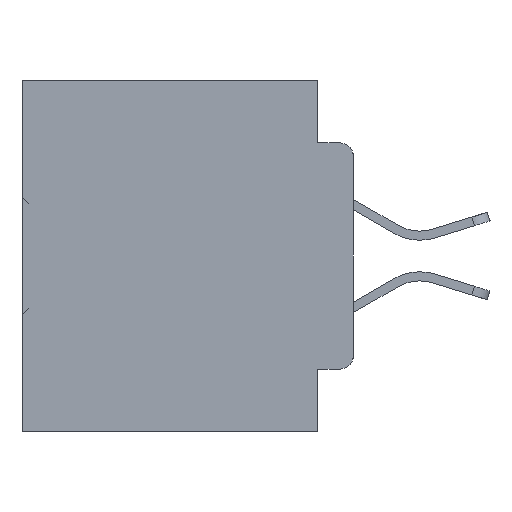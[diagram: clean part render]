
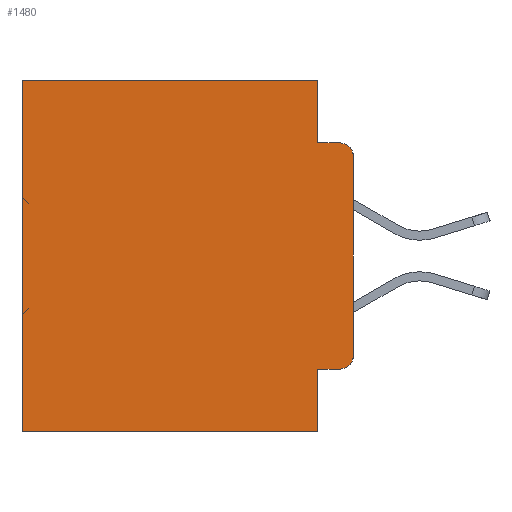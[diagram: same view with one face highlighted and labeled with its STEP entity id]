
A CAD part, left-side view. The second image highlights one B-rep face of the part: STEP entity #1480.
In plain terms, the highlighted planar face has unit normal (-1, 0, 0).
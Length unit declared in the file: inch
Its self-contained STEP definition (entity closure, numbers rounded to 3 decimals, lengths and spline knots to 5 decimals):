
#764 = CARTESIAN_POINT ( 'NONE',  ( 0.298, 0.02, -0.1085 ) ) ;
#821 = DIRECTION ( 'NONE',  ( 0., 1., 0. ) ) ;
#1219 = LINE ( 'NONE', #12970, #22932 ) ;
#1480 = ADVANCED_FACE ( 'NONE', ( #25447 ), #25645, .F. ) ;
#1769 = DIRECTION ( 'NONE',  ( 0., 0., -1. ) ) ;
#2023 = LINE ( 'NONE', #35336, #12925 ) ;
#2050 = CARTESIAN_POINT ( 'NONE',  ( 0.298, 0.051, -0.0885 ) ) ;
#2402 = CARTESIAN_POINT ( 'NONE',  ( 0.298, 0., -0.3915 ) ) ;
#3881 = VECTOR ( 'NONE', #14448, 39.37008 ) ;
#4180 = VECTOR ( 'NONE', #821, 39.37008 ) ;
#4468 = CARTESIAN_POINT ( 'NONE',  ( 0.298, 0.051, 0. ) ) ;
#5771 = LINE ( 'NONE', #36107, #29802 ) ;
#6191 = EDGE_CURVE ( 'NONE', #25917, #34526, #17168, .T. ) ;
#6485 = CARTESIAN_POINT ( 'NONE',  ( 0.298, 0.051, 0. ) ) ;
#7888 = ORIENTED_EDGE ( 'NONE', *, *, #6191, .F. ) ;
#8246 = VECTOR ( 'NONE', #15676, 39.37008 ) ;
#8309 = ORIENTED_EDGE ( 'NONE', *, *, #28857, .T. ) ;
#8771 = AXIS2_PLACEMENT_3D ( 'NONE', #764, #18760, #27748 ) ;
#8822 = AXIS2_PLACEMENT_3D ( 'NONE', #14044, #13656, #25971 ) ;
#8864 = LINE ( 'NONE', #30186, #8246 ) ;
#9851 = ORIENTED_EDGE ( 'NONE', *, *, #35419, .F. ) ;
#9973 = CARTESIAN_POINT ( 'NONE',  ( 0.298, 0.02, -0.0885 ) ) ;
#11407 = EDGE_CURVE ( 'NONE', #37395, #28947, #2023, .T. ) ;
#11568 = EDGE_CURVE ( 'NONE', #28137, #36050, #5771, .T. ) ;
#11791 = CARTESIAN_POINT ( 'NONE',  ( 0.298, 0., -0.1085 ) ) ;
#11933 = CIRCLE ( 'NONE', #8822, 0.02 ) ;
#12596 = DIRECTION ( 'NONE',  ( 0., -1., 0. ) ) ;
#12925 = VECTOR ( 'NONE', #29259, 39.37008 ) ;
#12970 = CARTESIAN_POINT ( 'NONE',  ( 0.298, 0.051, -0.4115 ) ) ;
#13656 = DIRECTION ( 'NONE',  ( -1., 0., 0. ) ) ;
#13900 = CARTESIAN_POINT ( 'NONE',  ( 0.298, 0.051, -0.4115 ) ) ;
#14044 = CARTESIAN_POINT ( 'NONE',  ( 0.298, 0.02, -0.3915 ) ) ;
#14448 = DIRECTION ( 'NONE',  ( 0., 0., -1. ) ) ;
#14636 = EDGE_LOOP ( 'NONE', ( #35437, #30565, #36561, #21337, #8309, #20432, #9851, #7888, #35831, #35888 ) ) ;
#15676 = DIRECTION ( 'NONE',  ( 0., 1., 0. ) ) ;
#15684 = LINE ( 'NONE', #36489, #4180 ) ;
#15830 = EDGE_CURVE ( 'NONE', #19145, #28137, #20118, .T. ) ;
#16073 = DIRECTION ( 'NONE',  ( 0., -1., 0. ) ) ;
#16640 = CARTESIAN_POINT ( 'NONE',  ( 0.298, 0., 0. ) ) ;
#17168 = LINE ( 'NONE', #25973, #3881 ) ;
#18032 = EDGE_CURVE ( 'NONE', #31664, #37157, #37619, .T. ) ;
#18760 = DIRECTION ( 'NONE',  ( -1., 0., 0. ) ) ;
#19145 = VERTEX_POINT ( 'NONE', #6485 ) ;
#20118 = LINE ( 'NONE', #4468, #26246 ) ;
#20432 = ORIENTED_EDGE ( 'NONE', *, *, #11407, .T. ) ;
#21337 = ORIENTED_EDGE ( 'NONE', *, *, #15830, .F. ) ;
#21567 = VERTEX_POINT ( 'NONE', #35968 ) ;
#21885 = CIRCLE ( 'NONE', #8771, 0.02 ) ;
#22683 = DIRECTION ( 'NONE',  ( 0., 0., -1. ) ) ;
#22932 = VECTOR ( 'NONE', #16073, 39.37008 ) ;
#25447 = FACE_OUTER_BOUND ( 'NONE', #14636, .T. ) ;
#25645 = PLANE ( 'NONE',  #27713 ) ;
#25917 = VERTEX_POINT ( 'NONE', #13900 ) ;
#25971 = DIRECTION ( 'NONE',  ( 0., 0., -1. ) ) ;
#25973 = CARTESIAN_POINT ( 'NONE',  ( 0.298, 0.051, 0. ) ) ;
#26246 = VECTOR ( 'NONE', #34632, 39.37008 ) ;
#26335 = EDGE_CURVE ( 'NONE', #31664, #36050, #21885, .T. ) ;
#27713 = AXIS2_PLACEMENT_3D ( 'NONE', #16640, #28597, #1769 ) ;
#27748 = DIRECTION ( 'NONE',  ( 0., 0., -1. ) ) ;
#28137 = VERTEX_POINT ( 'NONE', #2050 ) ;
#28597 = DIRECTION ( 'NONE',  ( 1., 0., 0. ) ) ;
#28803 = CARTESIAN_POINT ( 'NONE',  ( 0.298, 0.473, -0.5 ) ) ;
#28857 = EDGE_CURVE ( 'NONE', #19145, #37395, #15684, .T. ) ;
#28947 = VERTEX_POINT ( 'NONE', #28803 ) ;
#29259 = DIRECTION ( 'NONE',  ( 0., 0., -1. ) ) ;
#29802 = VECTOR ( 'NONE', #12596, 39.37008 ) ;
#30167 = EDGE_CURVE ( 'NONE', #25917, #21567, #1219, .T. ) ;
#30186 = CARTESIAN_POINT ( 'NONE',  ( 0.298, 0., -0.5 ) ) ;
#30317 = VECTOR ( 'NONE', #22683, 39.37008 ) ;
#30565 = ORIENTED_EDGE ( 'NONE', *, *, #26335, .T. ) ;
#31664 = VERTEX_POINT ( 'NONE', #11791 ) ;
#34526 = VERTEX_POINT ( 'NONE', #35455 ) ;
#34632 = DIRECTION ( 'NONE',  ( 0., 0., -1. ) ) ;
#35336 = CARTESIAN_POINT ( 'NONE',  ( 0.298, 0.473, 0. ) ) ;
#35419 = EDGE_CURVE ( 'NONE', #34526, #28947, #8864, .T. ) ;
#35437 = ORIENTED_EDGE ( 'NONE', *, *, #18032, .F. ) ;
#35455 = CARTESIAN_POINT ( 'NONE',  ( 0.298, 0.051, -0.5 ) ) ;
#35831 = ORIENTED_EDGE ( 'NONE', *, *, #30167, .T. ) ;
#35888 = ORIENTED_EDGE ( 'NONE', *, *, #36141, .T. ) ;
#35968 = CARTESIAN_POINT ( 'NONE',  ( 0.298, 0.02, -0.4115 ) ) ;
#36050 = VERTEX_POINT ( 'NONE', #9973 ) ;
#36107 = CARTESIAN_POINT ( 'NONE',  ( 0.298, 0.051, -0.0885 ) ) ;
#36141 = EDGE_CURVE ( 'NONE', #21567, #37157, #11933, .T. ) ;
#36489 = CARTESIAN_POINT ( 'NONE',  ( 0.298, 0., 0. ) ) ;
#36561 = ORIENTED_EDGE ( 'NONE', *, *, #11568, .F. ) ;
#36833 = CARTESIAN_POINT ( 'NONE',  ( 0.298, 0.473, 0. ) ) ;
#37045 = CARTESIAN_POINT ( 'NONE',  ( 0.298, 0., 0. ) ) ;
#37157 = VERTEX_POINT ( 'NONE', #2402 ) ;
#37395 = VERTEX_POINT ( 'NONE', #36833 ) ;
#37619 = LINE ( 'NONE', #37045, #30317 ) ;
